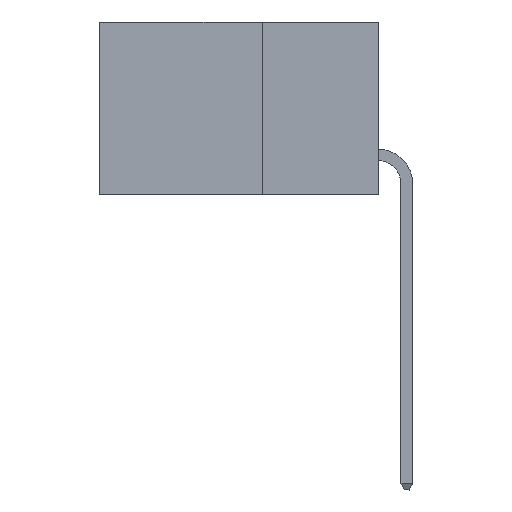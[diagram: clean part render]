
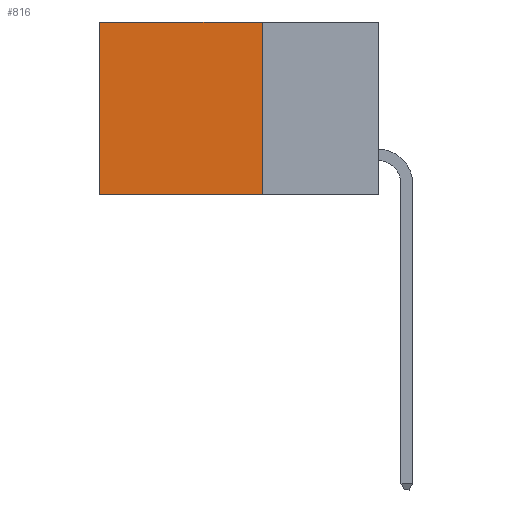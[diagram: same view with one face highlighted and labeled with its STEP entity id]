
A CAD part, left-side view. The second image highlights one B-rep face of the part: STEP entity #816.
In plain terms, the highlighted planar face has unit normal (-1, 0, 0).
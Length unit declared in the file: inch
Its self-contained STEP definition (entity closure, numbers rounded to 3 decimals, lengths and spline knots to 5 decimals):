
#642 = ORIENTED_EDGE ( 'NONE', *, *, #10254, .F. ) ;
#816 = ADVANCED_FACE ( 'NONE', ( #3615 ), #10398, .F. ) ;
#1242 = ORIENTED_EDGE ( 'NONE', *, *, #11370, .T. ) ;
#1257 = VECTOR ( 'NONE', #5215, 39.37008 ) ;
#1815 = CARTESIAN_POINT ( 'NONE',  ( 0.298, 0.6, -0.37 ) ) ;
#1854 = VERTEX_POINT ( 'NONE', #2651 ) ;
#1968 = VECTOR ( 'NONE', #13874, 39.37008 ) ;
#2651 = CARTESIAN_POINT ( 'NONE',  ( 0.298, 0.25, -0.37 ) ) ;
#3301 = DIRECTION ( 'NONE',  ( 0., 0., -1. ) ) ;
#3615 = FACE_OUTER_BOUND ( 'NONE', #7527, .T. ) ;
#4010 = LINE ( 'NONE', #14872, #1257 ) ;
#4469 = VECTOR ( 'NONE', #9410, 39.37008 ) ;
#5215 = DIRECTION ( 'NONE',  ( 0., 0., -1. ) ) ;
#5991 = VERTEX_POINT ( 'NONE', #1815 ) ;
#7047 = DIRECTION ( 'NONE',  ( 0., 0., -1. ) ) ;
#7278 = VERTEX_POINT ( 'NONE', #8581 ) ;
#7316 = CARTESIAN_POINT ( 'NONE',  ( 0.298, 0.25, 0. ) ) ;
#7365 = ORIENTED_EDGE ( 'NONE', *, *, #8268, .T. ) ;
#7527 = EDGE_LOOP ( 'NONE', ( #7365, #642, #17147, #1242 ) ) ;
#8052 = CARTESIAN_POINT ( 'NONE',  ( 0.298, 0.25, 0. ) ) ;
#8268 = EDGE_CURVE ( 'NONE', #7278, #5991, #4010, .T. ) ;
#8581 = CARTESIAN_POINT ( 'NONE',  ( 0.298, 0.6, 0. ) ) ;
#9410 = DIRECTION ( 'NONE',  ( 0., 1., 0. ) ) ;
#10254 = EDGE_CURVE ( 'NONE', #1854, #5991, #12931, .T. ) ;
#10393 = DIRECTION ( 'NONE',  ( 1., 0., 0. ) ) ;
#10398 = PLANE ( 'NONE',  #12487 ) ;
#11135 = CARTESIAN_POINT ( 'NONE',  ( 0.298, 0.25, -0.37 ) ) ;
#11370 = EDGE_CURVE ( 'NONE', #14109, #7278, #15451, .T. ) ;
#11554 = CARTESIAN_POINT ( 'NONE',  ( 0.298, 0.25, 0. ) ) ;
#11727 = EDGE_CURVE ( 'NONE', #14109, #1854, #11806, .T. ) ;
#11806 = LINE ( 'NONE', #11554, #15865 ) ;
#12487 = AXIS2_PLACEMENT_3D ( 'NONE', #7316, #10393, #7047 ) ;
#12931 = LINE ( 'NONE', #11135, #1968 ) ;
#13874 = DIRECTION ( 'NONE',  ( 0., 1., 0. ) ) ;
#14026 = CARTESIAN_POINT ( 'NONE',  ( 0.298, 0.25, 0. ) ) ;
#14109 = VERTEX_POINT ( 'NONE', #14026 ) ;
#14872 = CARTESIAN_POINT ( 'NONE',  ( 0.298, 0.6, 0. ) ) ;
#15451 = LINE ( 'NONE', #8052, #4469 ) ;
#15865 = VECTOR ( 'NONE', #3301, 39.37008 ) ;
#17147 = ORIENTED_EDGE ( 'NONE', *, *, #11727, .F. ) ;
